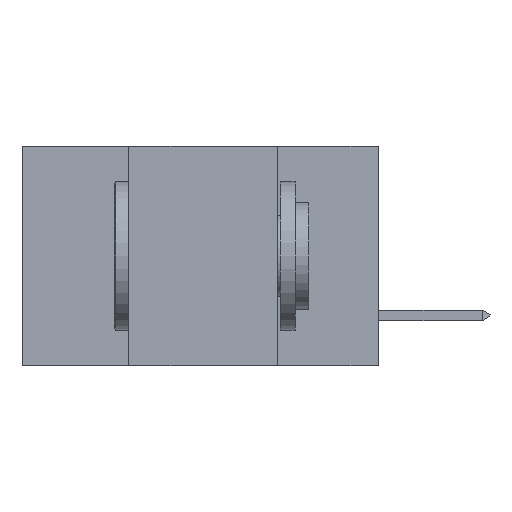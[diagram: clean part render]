
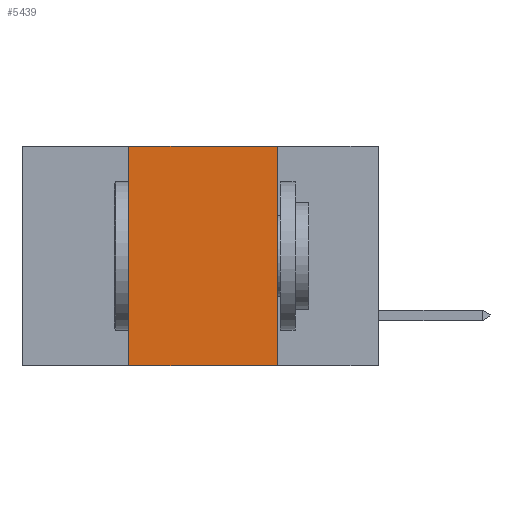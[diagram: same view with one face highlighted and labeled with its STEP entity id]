
A CAD part, left-side view. The second image highlights one B-rep face of the part: STEP entity #5439.
In plain terms, the highlighted planar face has unit normal (-1, 0, 0).
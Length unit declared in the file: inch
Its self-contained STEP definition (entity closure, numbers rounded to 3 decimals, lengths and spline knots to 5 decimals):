
#244 = VECTOR ( 'NONE', #4736, 39.37008 ) ;
#463 = LINE ( 'NONE', #4532, #3005 ) ;
#693 = EDGE_LOOP ( 'NONE', ( #6550, #929, #9186, #10163 ) ) ;
#929 = ORIENTED_EDGE ( 'NONE', *, *, #5240, .F. ) ;
#1132 = CARTESIAN_POINT ( 'NONE',  ( 0., 0.42, -0.37 ) ) ;
#2320 = PLANE ( 'NONE',  #2832 ) ;
#2760 = LINE ( 'NONE', #7032, #4054 ) ;
#2832 = AXIS2_PLACEMENT_3D ( 'NONE', #5606, #3958, #9047 ) ;
#2876 = CARTESIAN_POINT ( 'NONE',  ( 0., 0.17, -0.37 ) ) ;
#3005 = VECTOR ( 'NONE', #7314, 39.37008 ) ;
#3777 = VERTEX_POINT ( 'NONE', #5367 ) ;
#3958 = DIRECTION ( 'NONE',  ( 1., 0., 0. ) ) ;
#3968 = CARTESIAN_POINT ( 'NONE',  ( 0., 0.42, 0. ) ) ;
#4054 = VECTOR ( 'NONE', #8031, 39.37008 ) ;
#4532 = CARTESIAN_POINT ( 'NONE',  ( 0., 0.6, -0.37 ) ) ;
#4736 = DIRECTION ( 'NONE',  ( 0., 0., -1. ) ) ;
#5240 = EDGE_CURVE ( 'NONE', #9634, #3777, #2760, .T. ) ;
#5367 = CARTESIAN_POINT ( 'NONE',  ( 0., 0.17, 0. ) ) ;
#5439 = ADVANCED_FACE ( 'NONE', ( #6688 ), #2320, .F. ) ;
#5606 = CARTESIAN_POINT ( 'NONE',  ( 0., 0.6, 0. ) ) ;
#6550 = ORIENTED_EDGE ( 'NONE', *, *, #10664, .F. ) ;
#6629 = LINE ( 'NONE', #10053, #7674 ) ;
#6688 = FACE_OUTER_BOUND ( 'NONE', #693, .T. ) ;
#6946 = DIRECTION ( 'NONE',  ( 0., 0., 1. ) ) ;
#7032 = CARTESIAN_POINT ( 'NONE',  ( 0., 0.6, 0. ) ) ;
#7047 = CARTESIAN_POINT ( 'NONE',  ( 0., 0.17, -0.37 ) ) ;
#7314 = DIRECTION ( 'NONE',  ( 0., -1., 0. ) ) ;
#7674 = VECTOR ( 'NONE', #6946, 39.37008 ) ;
#8031 = DIRECTION ( 'NONE',  ( 0., -1., 0. ) ) ;
#8284 = EDGE_CURVE ( 'NONE', #9576, #9421, #463, .T. ) ;
#8968 = EDGE_CURVE ( 'NONE', #9576, #9634, #6629, .T. ) ;
#9047 = DIRECTION ( 'NONE',  ( 0., 0., -1. ) ) ;
#9186 = ORIENTED_EDGE ( 'NONE', *, *, #8968, .F. ) ;
#9421 = VERTEX_POINT ( 'NONE', #7047 ) ;
#9576 = VERTEX_POINT ( 'NONE', #1132 ) ;
#9634 = VERTEX_POINT ( 'NONE', #3968 ) ;
#9713 = LINE ( 'NONE', #2876, #244 ) ;
#10053 = CARTESIAN_POINT ( 'NONE',  ( 0., 0.42, -0.37 ) ) ;
#10163 = ORIENTED_EDGE ( 'NONE', *, *, #8284, .T. ) ;
#10664 = EDGE_CURVE ( 'NONE', #3777, #9421, #9713, .T. ) ;
